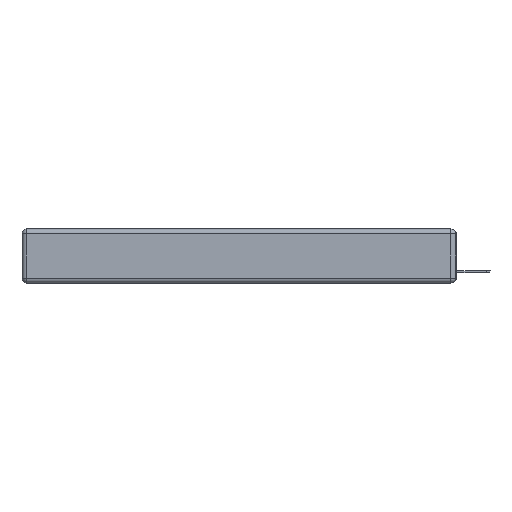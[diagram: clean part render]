
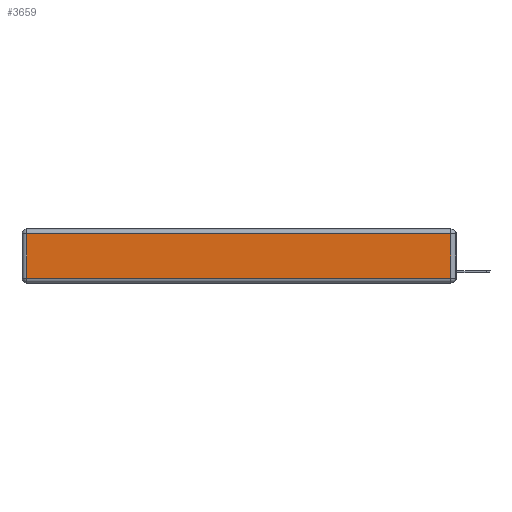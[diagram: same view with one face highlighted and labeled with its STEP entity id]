
A CAD part, left-side view. The second image highlights one B-rep face of the part: STEP entity #3659.
In plain terms, the highlighted planar face has unit normal (-1, 0, 0).
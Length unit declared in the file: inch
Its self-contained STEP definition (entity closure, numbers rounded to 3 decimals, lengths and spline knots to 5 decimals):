
#233 = CARTESIAN_POINT ( 'NONE',  ( 0., 0.03, -0.343 ) ) ;
#1228 = LINE ( 'NONE', #10831, #8057 ) ;
#1416 = VECTOR ( 'NONE', #5334, 39.37008 ) ;
#1999 = CARTESIAN_POINT ( 'NONE',  ( 0., 2.72, -0.313 ) ) ;
#2162 = CARTESIAN_POINT ( 'NONE',  ( 0., 2.72, -0.03 ) ) ;
#3017 = EDGE_LOOP ( 'NONE', ( #4472, #8864, #10622, #10288 ) ) ;
#3638 = DIRECTION ( 'NONE',  ( 0., 1., 0. ) ) ;
#3659 = ADVANCED_FACE ( 'NONE', ( #12664 ), #5124, .T. ) ;
#3755 = EDGE_CURVE ( 'NONE', #4469, #12194, #11807, .T. ) ;
#3771 = CARTESIAN_POINT ( 'NONE',  ( 0., 2.75, -0.03 ) ) ;
#4085 = CARTESIAN_POINT ( 'NONE',  ( 0., 0., -0.343 ) ) ;
#4469 = VERTEX_POINT ( 'NONE', #4826 ) ;
#4472 = ORIENTED_EDGE ( 'NONE', *, *, #13110, .T. ) ;
#4826 = CARTESIAN_POINT ( 'NONE',  ( 0., 0.03, -0.313 ) ) ;
#5124 = PLANE ( 'NONE',  #5198 ) ;
#5198 = AXIS2_PLACEMENT_3D ( 'NONE', #4085, #9328, #13771 ) ;
#5334 = DIRECTION ( 'NONE',  ( 0., 0., 1. ) ) ;
#5931 = LINE ( 'NONE', #3771, #10808 ) ;
#6008 = CARTESIAN_POINT ( 'NONE',  ( 0., 0., -0.313 ) ) ;
#6082 = DIRECTION ( 'NONE',  ( 0., -1., 0. ) ) ;
#6533 = DIRECTION ( 'NONE',  ( 0., 0., -1. ) ) ;
#7538 = EDGE_CURVE ( 'NONE', #12194, #9912, #5931, .T. ) ;
#7925 = CARTESIAN_POINT ( 'NONE',  ( 0., 0.03, -0.03 ) ) ;
#8057 = VECTOR ( 'NONE', #6533, 39.37008 ) ;
#8251 = LINE ( 'NONE', #6008, #13406 ) ;
#8864 = ORIENTED_EDGE ( 'NONE', *, *, #3755, .T. ) ;
#9328 = DIRECTION ( 'NONE',  ( -1., 0., 0. ) ) ;
#9912 = VERTEX_POINT ( 'NONE', #2162 ) ;
#10288 = ORIENTED_EDGE ( 'NONE', *, *, #11945, .T. ) ;
#10622 = ORIENTED_EDGE ( 'NONE', *, *, #7538, .T. ) ;
#10668 = VERTEX_POINT ( 'NONE', #1999 ) ;
#10808 = VECTOR ( 'NONE', #3638, 39.37008 ) ;
#10831 = CARTESIAN_POINT ( 'NONE',  ( 0., 2.72, -0.343 ) ) ;
#11807 = LINE ( 'NONE', #233, #1416 ) ;
#11945 = EDGE_CURVE ( 'NONE', #9912, #10668, #1228, .T. ) ;
#12194 = VERTEX_POINT ( 'NONE', #7925 ) ;
#12664 = FACE_OUTER_BOUND ( 'NONE', #3017, .T. ) ;
#13110 = EDGE_CURVE ( 'NONE', #10668, #4469, #8251, .T. ) ;
#13406 = VECTOR ( 'NONE', #6082, 39.37008 ) ;
#13771 = DIRECTION ( 'NONE',  ( 0., 0., 1. ) ) ;
